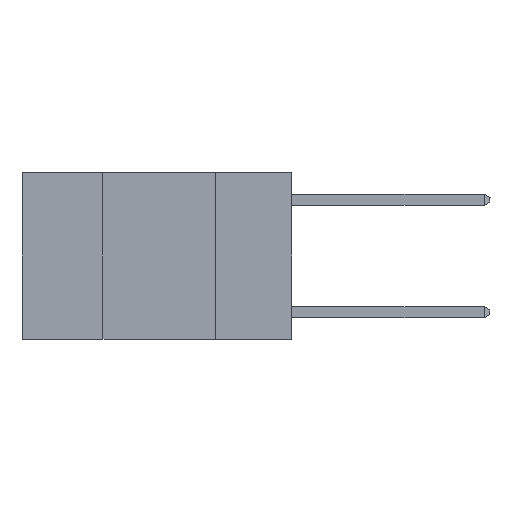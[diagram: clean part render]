
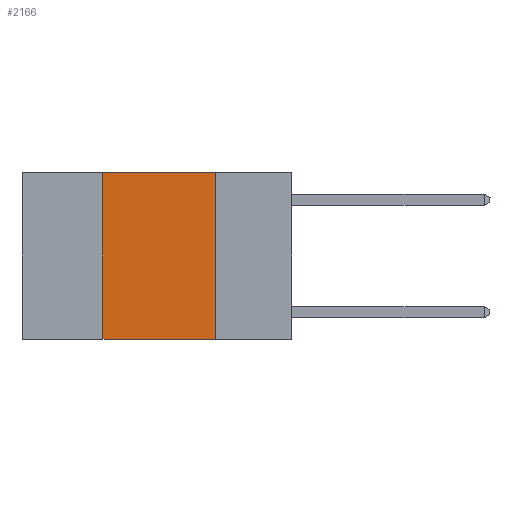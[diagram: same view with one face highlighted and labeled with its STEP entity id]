
A CAD part, left-side view. The second image highlights one B-rep face of the part: STEP entity #2166.
In plain terms, the highlighted planar face has unit normal (-1, 0, 0).
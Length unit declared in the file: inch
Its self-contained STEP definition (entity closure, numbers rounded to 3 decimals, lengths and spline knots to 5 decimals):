
#295 = DIRECTION ( 'NONE',  ( 0., 0., 1. ) ) ;
#502 = VECTOR ( 'NONE', #4362, 39.37008 ) ;
#805 = CARTESIAN_POINT ( 'NONE',  ( 0., 0.42, -0.37 ) ) ;
#919 = VERTEX_POINT ( 'NONE', #7705 ) ;
#1709 = VERTEX_POINT ( 'NONE', #805 ) ;
#1928 = EDGE_LOOP ( 'NONE', ( #7305, #6818, #4526, #2681 ) ) ;
#1951 = VECTOR ( 'NONE', #4801, 39.37008 ) ;
#2166 = ADVANCED_FACE ( 'NONE', ( #6440 ), #2398, .F. ) ;
#2197 = EDGE_CURVE ( 'NONE', #1709, #3999, #5117, .T. ) ;
#2311 = LINE ( 'NONE', #5073, #5284 ) ;
#2398 = PLANE ( 'NONE',  #5655 ) ;
#2681 = ORIENTED_EDGE ( 'NONE', *, *, #4418, .T. ) ;
#3013 = LINE ( 'NONE', #5734, #502 ) ;
#3030 = CARTESIAN_POINT ( 'NONE',  ( 0., 0.6, 0. ) ) ;
#3182 = VECTOR ( 'NONE', #295, 39.37008 ) ;
#3599 = DIRECTION ( 'NONE',  ( 0., 0., -1. ) ) ;
#3683 = CARTESIAN_POINT ( 'NONE',  ( 0., 0.42, 0. ) ) ;
#3776 = EDGE_CURVE ( 'NONE', #3999, #5366, #4858, .T. ) ;
#3999 = VERTEX_POINT ( 'NONE', #5930 ) ;
#4362 = DIRECTION ( 'NONE',  ( 0., -1., 0. ) ) ;
#4418 = EDGE_CURVE ( 'NONE', #1709, #919, #3013, .T. ) ;
#4526 = ORIENTED_EDGE ( 'NONE', *, *, #2197, .F. ) ;
#4801 = DIRECTION ( 'NONE',  ( 0., -1., 0. ) ) ;
#4858 = LINE ( 'NONE', #7488, #1951 ) ;
#5073 = CARTESIAN_POINT ( 'NONE',  ( 0., 0.17, 0. ) ) ;
#5117 = LINE ( 'NONE', #3683, #3182 ) ;
#5284 = VECTOR ( 'NONE', #7797, 39.37008 ) ;
#5366 = VERTEX_POINT ( 'NONE', #7677 ) ;
#5655 = AXIS2_PLACEMENT_3D ( 'NONE', #3030, #7068, #3599 ) ;
#5734 = CARTESIAN_POINT ( 'NONE',  ( 0., 0.6, -0.37 ) ) ;
#5930 = CARTESIAN_POINT ( 'NONE',  ( 0., 0.42, 0. ) ) ;
#5972 = EDGE_CURVE ( 'NONE', #5366, #919, #2311, .T. ) ;
#6440 = FACE_OUTER_BOUND ( 'NONE', #1928, .T. ) ;
#6818 = ORIENTED_EDGE ( 'NONE', *, *, #3776, .F. ) ;
#7068 = DIRECTION ( 'NONE',  ( 1., 0., 0. ) ) ;
#7305 = ORIENTED_EDGE ( 'NONE', *, *, #5972, .F. ) ;
#7488 = CARTESIAN_POINT ( 'NONE',  ( 0., 0.6, 0. ) ) ;
#7677 = CARTESIAN_POINT ( 'NONE',  ( 0., 0.17, 0. ) ) ;
#7705 = CARTESIAN_POINT ( 'NONE',  ( 0., 0.17, -0.37 ) ) ;
#7797 = DIRECTION ( 'NONE',  ( 0., 0., -1. ) ) ;
